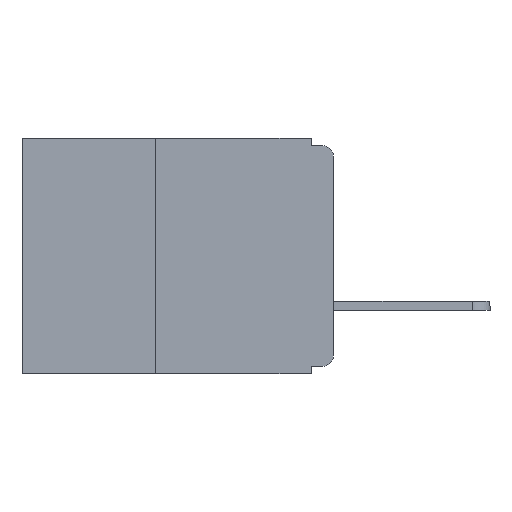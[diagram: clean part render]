
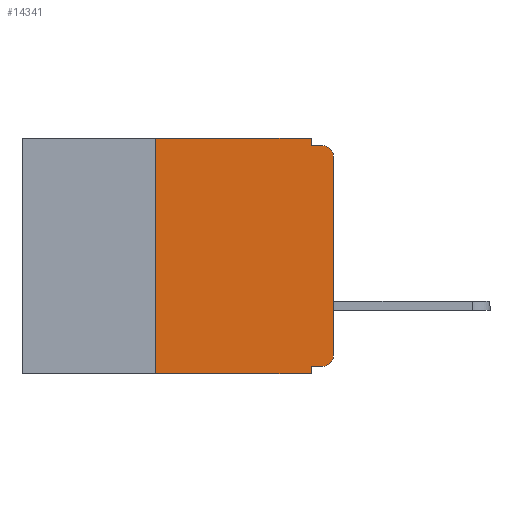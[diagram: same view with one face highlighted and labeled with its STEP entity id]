
A CAD part, left-side view. The second image highlights one B-rep face of the part: STEP entity #14341.
In plain terms, the highlighted planar face has unit normal (-1, 0, 0).
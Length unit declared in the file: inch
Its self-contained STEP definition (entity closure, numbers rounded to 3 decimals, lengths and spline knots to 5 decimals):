
#7 = DIRECTION ( 'NONE',  ( 0., -1., 0. ) ) ;
#419 = LINE ( 'NONE', #2528, #12652 ) ;
#451 = VERTEX_POINT ( 'NONE', #13265 ) ;
#732 = LINE ( 'NONE', #19650, #18646 ) ;
#1200 = DIRECTION ( 'NONE',  ( 0., 0., -1. ) ) ;
#1480 = LINE ( 'NONE', #21883, #19369 ) ;
#1592 = EDGE_CURVE ( 'NONE', #21362, #2586, #419, .T. ) ;
#1764 = DIRECTION ( 'NONE',  ( 0., 0., -1. ) ) ;
#2346 = EDGE_CURVE ( 'NONE', #2586, #451, #1480, .T. ) ;
#2390 = DIRECTION ( 'NONE',  ( 0., -1., 0. ) ) ;
#2528 = CARTESIAN_POINT ( 'NONE',  ( 0., 0., -0.32 ) ) ;
#2586 = VERTEX_POINT ( 'NONE', #20884 ) ;
#3320 = EDGE_CURVE ( 'NONE', #12061, #6475, #732, .T. ) ;
#3436 = VERTEX_POINT ( 'NONE', #4374 ) ;
#3625 = DIRECTION ( 'NONE',  ( 0., -1., 0. ) ) ;
#3922 = ORIENTED_EDGE ( 'NONE', *, *, #2346, .F. ) ;
#4284 = ORIENTED_EDGE ( 'NONE', *, *, #13811, .T. ) ;
#4374 = CARTESIAN_POINT ( 'NONE',  ( 0., 0., -0.025 ) ) ;
#4436 = CARTESIAN_POINT ( 'NONE',  ( 0., 0.015, -0.025 ) ) ;
#4581 = VECTOR ( 'NONE', #18118, 39.37008 ) ;
#4678 = CARTESIAN_POINT ( 'NONE',  ( 0., 0.25, 0. ) ) ;
#4908 = VERTEX_POINT ( 'NONE', #6049 ) ;
#4958 = CIRCLE ( 'NONE', #7619, 0.015 ) ;
#5252 = VERTEX_POINT ( 'NONE', #17286 ) ;
#5501 = CIRCLE ( 'NONE', #17644, 0.015 ) ;
#5536 = ORIENTED_EDGE ( 'NONE', *, *, #19880, .T. ) ;
#5604 = PLANE ( 'NONE',  #7820 ) ;
#5937 = VECTOR ( 'NONE', #7, 39.37008 ) ;
#6049 = CARTESIAN_POINT ( 'NONE',  ( 0., 0.25, -0.33 ) ) ;
#6060 = CARTESIAN_POINT ( 'NONE',  ( 0., 0.25, -0.33 ) ) ;
#6132 = VERTEX_POINT ( 'NONE', #8078 ) ;
#6475 = VERTEX_POINT ( 'NONE', #19404 ) ;
#6677 = ORIENTED_EDGE ( 'NONE', *, *, #3320, .F. ) ;
#7304 = DIRECTION ( 'NONE',  ( 1., 0., 0. ) ) ;
#7619 = AXIS2_PLACEMENT_3D ( 'NONE', #4436, #12157, #1764 ) ;
#7820 = AXIS2_PLACEMENT_3D ( 'NONE', #14216, #7304, #19399 ) ;
#7971 = CARTESIAN_POINT ( 'NONE',  ( 0., 0.015, -0.305 ) ) ;
#8078 = CARTESIAN_POINT ( 'NONE',  ( 0., 0.031, 0. ) ) ;
#8716 = DIRECTION ( 'NONE',  ( 0., 0., -1. ) ) ;
#9195 = LINE ( 'NONE', #19909, #4581 ) ;
#9708 = DIRECTION ( 'NONE',  ( 0., 0., -1. ) ) ;
#10373 = VECTOR ( 'NONE', #3625, 39.37008 ) ;
#10457 = CARTESIAN_POINT ( 'NONE',  ( 0., 0.031, 0. ) ) ;
#10515 = LINE ( 'NONE', #19115, #5937 ) ;
#10688 = EDGE_CURVE ( 'NONE', #3436, #6475, #4958, .T. ) ;
#10882 = CARTESIAN_POINT ( 'NONE',  ( 0., 0.031, -0.01 ) ) ;
#11019 = EDGE_CURVE ( 'NONE', #21362, #5252, #5501, .T. ) ;
#12061 = VERTEX_POINT ( 'NONE', #10882 ) ;
#12157 = DIRECTION ( 'NONE',  ( -1., 0., 0. ) ) ;
#12174 = EDGE_CURVE ( 'NONE', #4908, #13985, #17327, .T. ) ;
#12652 = VECTOR ( 'NONE', #14601, 39.37008 ) ;
#13154 = EDGE_CURVE ( 'NONE', #6132, #12061, #19461, .T. ) ;
#13265 = CARTESIAN_POINT ( 'NONE',  ( 0., 0.031, -0.33 ) ) ;
#13630 = ORIENTED_EDGE ( 'NONE', *, *, #1592, .F. ) ;
#13811 = EDGE_CURVE ( 'NONE', #4908, #451, #10515, .T. ) ;
#13985 = VERTEX_POINT ( 'NONE', #4678 ) ;
#14216 = CARTESIAN_POINT ( 'NONE',  ( 0., 0.437, 0. ) ) ;
#14341 = ADVANCED_FACE ( 'NONE', ( #21829 ), #5604, .F. ) ;
#14601 = DIRECTION ( 'NONE',  ( 0., 1., 0. ) ) ;
#14869 = VECTOR ( 'NONE', #8716, 39.37008 ) ;
#15196 = ORIENTED_EDGE ( 'NONE', *, *, #10688, .T. ) ;
#16013 = CARTESIAN_POINT ( 'NONE',  ( 0., 0.015, -0.32 ) ) ;
#17286 = CARTESIAN_POINT ( 'NONE',  ( 0., 0., -0.305 ) ) ;
#17327 = LINE ( 'NONE', #6060, #22441 ) ;
#17560 = CARTESIAN_POINT ( 'NONE',  ( 0., 0.437, 0. ) ) ;
#17644 = AXIS2_PLACEMENT_3D ( 'NONE', #7971, #20062, #9708 ) ;
#17703 = EDGE_CURVE ( 'NONE', #13985, #6132, #19032, .T. ) ;
#18118 = DIRECTION ( 'NONE',  ( 0., 0., 1. ) ) ;
#18144 = DIRECTION ( 'NONE',  ( 0., 0., 1. ) ) ;
#18646 = VECTOR ( 'NONE', #2390, 39.37008 ) ;
#19032 = LINE ( 'NONE', #17560, #10373 ) ;
#19115 = CARTESIAN_POINT ( 'NONE',  ( 0., 0.437, -0.33 ) ) ;
#19273 = ORIENTED_EDGE ( 'NONE', *, *, #11019, .T. ) ;
#19369 = VECTOR ( 'NONE', #1200, 39.37008 ) ;
#19399 = DIRECTION ( 'NONE',  ( 0., 0., -1. ) ) ;
#19403 = ORIENTED_EDGE ( 'NONE', *, *, #13154, .F. ) ;
#19404 = CARTESIAN_POINT ( 'NONE',  ( 0., 0.015, -0.01 ) ) ;
#19461 = LINE ( 'NONE', #10457, #14869 ) ;
#19650 = CARTESIAN_POINT ( 'NONE',  ( 0., 0., -0.01 ) ) ;
#19880 = EDGE_CURVE ( 'NONE', #5252, #3436, #9195, .T. ) ;
#19909 = CARTESIAN_POINT ( 'NONE',  ( 0., 0., 0. ) ) ;
#19915 = EDGE_LOOP ( 'NONE', ( #5536, #15196, #6677, #19403, #20349, #22414, #4284, #3922, #13630, #19273 ) ) ;
#20062 = DIRECTION ( 'NONE',  ( -1., 0., 0. ) ) ;
#20349 = ORIENTED_EDGE ( 'NONE', *, *, #17703, .F. ) ;
#20884 = CARTESIAN_POINT ( 'NONE',  ( 0., 0.031, -0.32 ) ) ;
#21362 = VERTEX_POINT ( 'NONE', #16013 ) ;
#21829 = FACE_OUTER_BOUND ( 'NONE', #19915, .T. ) ;
#21883 = CARTESIAN_POINT ( 'NONE',  ( 0., 0.031, -0.33 ) ) ;
#22414 = ORIENTED_EDGE ( 'NONE', *, *, #12174, .F. ) ;
#22441 = VECTOR ( 'NONE', #18144, 39.37008 ) ;
